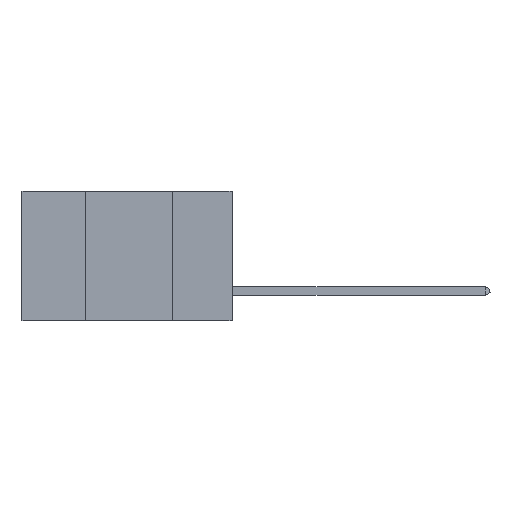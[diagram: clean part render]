
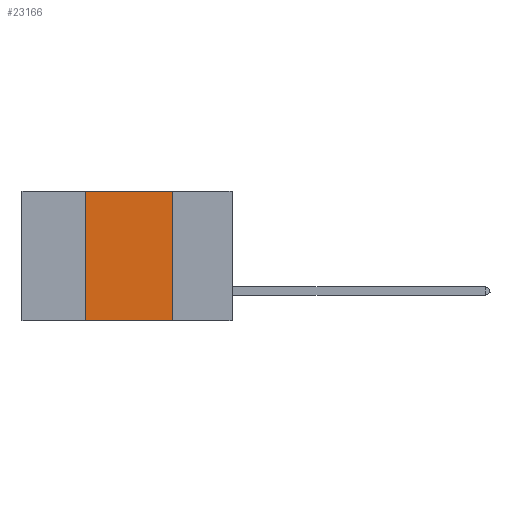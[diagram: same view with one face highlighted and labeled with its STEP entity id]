
A CAD part, left-side view. The second image highlights one B-rep face of the part: STEP entity #23166.
In plain terms, the highlighted planar face has unit normal (-1, 0, 0).
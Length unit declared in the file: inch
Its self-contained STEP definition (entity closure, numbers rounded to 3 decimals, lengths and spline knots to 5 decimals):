
#1925 = LINE ( 'NONE', #14165, #24359 ) ;
#2436 = CARTESIAN_POINT ( 'NONE',  ( 0., 0.6, 0. ) ) ;
#4281 = CARTESIAN_POINT ( 'NONE',  ( 0., 0.42, 0. ) ) ;
#5000 = VERTEX_POINT ( 'NONE', #37676 ) ;
#6962 = VERTEX_POINT ( 'NONE', #17256 ) ;
#8484 = VECTOR ( 'NONE', #20215, 39.37008 ) ;
#8706 = LINE ( 'NONE', #24504, #10559 ) ;
#9594 = DIRECTION ( 'NONE',  ( 0., -1., 0. ) ) ;
#10494 = FACE_OUTER_BOUND ( 'NONE', #29180, .T. ) ;
#10559 = VECTOR ( 'NONE', #9594, 39.37008 ) ;
#10857 = VERTEX_POINT ( 'NONE', #18833 ) ;
#12577 = ORIENTED_EDGE ( 'NONE', *, *, #30190, .F. ) ;
#14165 = CARTESIAN_POINT ( 'NONE',  ( 0., 0.17, 0. ) ) ;
#17256 = CARTESIAN_POINT ( 'NONE',  ( 0., 0.42, -0.37 ) ) ;
#17715 = EDGE_CURVE ( 'NONE', #5000, #10857, #8706, .T. ) ;
#18833 = CARTESIAN_POINT ( 'NONE',  ( 0., 0.17, 0. ) ) ;
#19969 = DIRECTION ( 'NONE',  ( 0., 0., -1. ) ) ;
#20071 = VERTEX_POINT ( 'NONE', #34188 ) ;
#20215 = DIRECTION ( 'NONE',  ( 0., 0., 1. ) ) ;
#21436 = AXIS2_PLACEMENT_3D ( 'NONE', #2436, #31504, #19969 ) ;
#23015 = ORIENTED_EDGE ( 'NONE', *, *, #34162, .F. ) ;
#23166 = ADVANCED_FACE ( 'NONE', ( #10494 ), #25625, .F. ) ;
#24119 = LINE ( 'NONE', #4281, #8484 ) ;
#24359 = VECTOR ( 'NONE', #28918, 39.37008 ) ;
#24396 = DIRECTION ( 'NONE',  ( 0., -1., 0. ) ) ;
#24504 = CARTESIAN_POINT ( 'NONE',  ( 0., 0.6, 0. ) ) ;
#25625 = PLANE ( 'NONE',  #21436 ) ;
#27767 = LINE ( 'NONE', #33225, #37006 ) ;
#28918 = DIRECTION ( 'NONE',  ( 0., 0., -1. ) ) ;
#29180 = EDGE_LOOP ( 'NONE', ( #23015, #31731, #12577, #31459 ) ) ;
#30084 = EDGE_CURVE ( 'NONE', #6962, #20071, #27767, .T. ) ;
#30190 = EDGE_CURVE ( 'NONE', #6962, #5000, #24119, .T. ) ;
#31459 = ORIENTED_EDGE ( 'NONE', *, *, #30084, .T. ) ;
#31504 = DIRECTION ( 'NONE',  ( 1., 0., 0. ) ) ;
#31731 = ORIENTED_EDGE ( 'NONE', *, *, #17715, .F. ) ;
#33225 = CARTESIAN_POINT ( 'NONE',  ( 0., 0.6, -0.37 ) ) ;
#34162 = EDGE_CURVE ( 'NONE', #10857, #20071, #1925, .T. ) ;
#34188 = CARTESIAN_POINT ( 'NONE',  ( 0., 0.17, -0.37 ) ) ;
#37006 = VECTOR ( 'NONE', #24396, 39.37008 ) ;
#37676 = CARTESIAN_POINT ( 'NONE',  ( 0., 0.42, 0. ) ) ;
